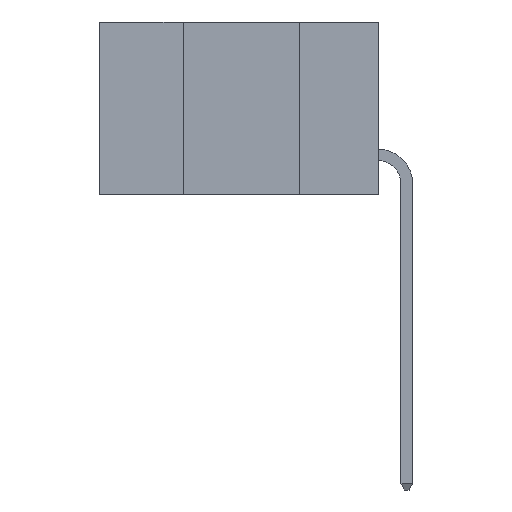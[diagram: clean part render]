
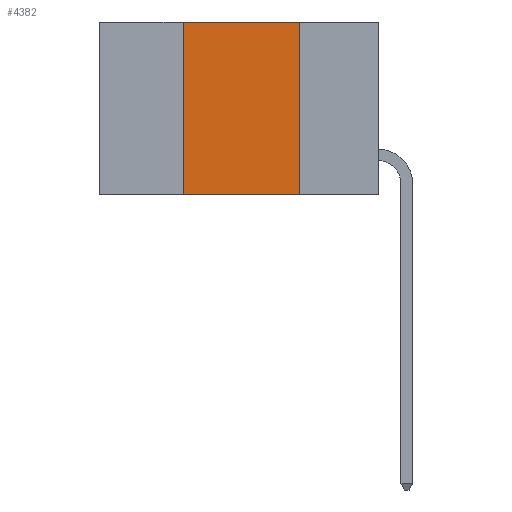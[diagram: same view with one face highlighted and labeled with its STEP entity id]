
A CAD part, left-side view. The second image highlights one B-rep face of the part: STEP entity #4382.
In plain terms, the highlighted planar face has unit normal (-1, 0, 0).
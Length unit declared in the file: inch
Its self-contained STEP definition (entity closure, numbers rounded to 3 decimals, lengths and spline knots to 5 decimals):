
#866 = EDGE_CURVE ( 'NONE', #18922, #11898, #16435, .T. ) ;
#1530 = DIRECTION ( 'NONE',  ( 0., -1., 0. ) ) ;
#1733 = DIRECTION ( 'NONE',  ( 0., 0., -1. ) ) ;
#1787 = DIRECTION ( 'NONE',  ( 1., 0., 0. ) ) ;
#1810 = PLANE ( 'NONE',  #5848 ) ;
#1910 = CARTESIAN_POINT ( 'NONE',  ( 0., 0.6, -0.37 ) ) ;
#1971 = VECTOR ( 'NONE', #1530, 39.37008 ) ;
#2068 = CARTESIAN_POINT ( 'NONE',  ( 0., 0.6, 0. ) ) ;
#3997 = CARTESIAN_POINT ( 'NONE',  ( 0., 0.17, 0. ) ) ;
#4382 = ADVANCED_FACE ( 'NONE', ( #19918 ), #1810, .F. ) ;
#4547 = CARTESIAN_POINT ( 'NONE',  ( 0., 0.42, -0.37 ) ) ;
#4952 = ORIENTED_EDGE ( 'NONE', *, *, #866, .F. ) ;
#5348 = CARTESIAN_POINT ( 'NONE',  ( 0., 0.42, 0. ) ) ;
#5683 = EDGE_CURVE ( 'NONE', #18922, #12344, #6747, .T. ) ;
#5848 = AXIS2_PLACEMENT_3D ( 'NONE', #2068, #1787, #1733 ) ;
#6747 = LINE ( 'NONE', #1910, #1971 ) ;
#6918 = EDGE_CURVE ( 'NONE', #11898, #10713, #9984, .T. ) ;
#7123 = CARTESIAN_POINT ( 'NONE',  ( 0., 0.6, 0. ) ) ;
#8181 = LINE ( 'NONE', #13442, #12845 ) ;
#9775 = EDGE_CURVE ( 'NONE', #10713, #12344, #8181, .T. ) ;
#9984 = LINE ( 'NONE', #7123, #14104 ) ;
#10713 = VERTEX_POINT ( 'NONE', #3997 ) ;
#11533 = ORIENTED_EDGE ( 'NONE', *, *, #9775, .F. ) ;
#11755 = VECTOR ( 'NONE', #15928, 39.37008 ) ;
#11898 = VERTEX_POINT ( 'NONE', #5348 ) ;
#12019 = CARTESIAN_POINT ( 'NONE',  ( 0., 0.17, -0.37 ) ) ;
#12344 = VERTEX_POINT ( 'NONE', #12019 ) ;
#12845 = VECTOR ( 'NONE', #22117, 39.37008 ) ;
#13442 = CARTESIAN_POINT ( 'NONE',  ( 0., 0.17, -0.37 ) ) ;
#13849 = ORIENTED_EDGE ( 'NONE', *, *, #6918, .F. ) ;
#14104 = VECTOR ( 'NONE', #17618, 39.37008 ) ;
#15772 = CARTESIAN_POINT ( 'NONE',  ( 0., 0.42, -0.37 ) ) ;
#15928 = DIRECTION ( 'NONE',  ( 0., 0., 1. ) ) ;
#16435 = LINE ( 'NONE', #15772, #11755 ) ;
#17618 = DIRECTION ( 'NONE',  ( 0., -1., 0. ) ) ;
#18922 = VERTEX_POINT ( 'NONE', #4547 ) ;
#18993 = EDGE_LOOP ( 'NONE', ( #11533, #13849, #4952, #22304 ) ) ;
#19918 = FACE_OUTER_BOUND ( 'NONE', #18993, .T. ) ;
#22117 = DIRECTION ( 'NONE',  ( 0., 0., -1. ) ) ;
#22304 = ORIENTED_EDGE ( 'NONE', *, *, #5683, .T. ) ;
